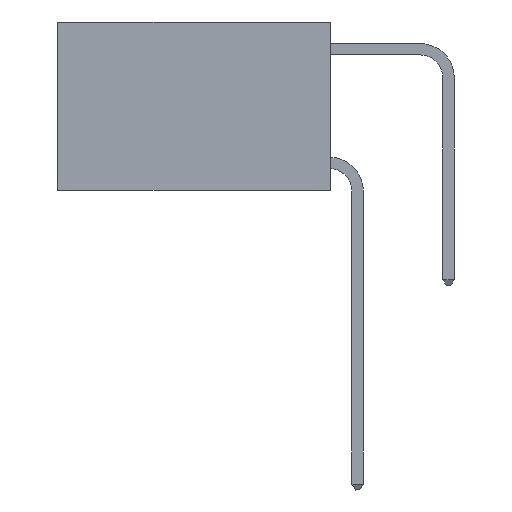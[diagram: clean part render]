
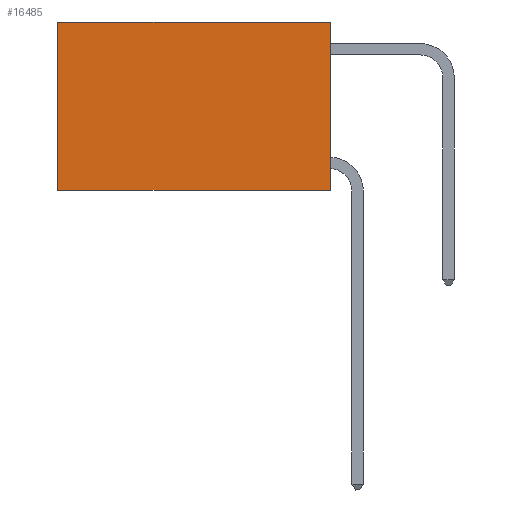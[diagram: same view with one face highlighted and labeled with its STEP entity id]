
A CAD part, left-side view. The second image highlights one B-rep face of the part: STEP entity #16485.
In plain terms, the highlighted planar face has unit normal (-1, 0, 0).
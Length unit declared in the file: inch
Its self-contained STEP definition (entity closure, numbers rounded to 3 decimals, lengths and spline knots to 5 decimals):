
#1286 = LINE ( 'NONE', #7868, #14220 ) ;
#1304 = PLANE ( 'NONE',  #7939 ) ;
#2613 = ORIENTED_EDGE ( 'NONE', *, *, #19795, .T. ) ;
#2713 = VERTEX_POINT ( 'NONE', #18414 ) ;
#2981 = FACE_OUTER_BOUND ( 'NONE', #11656, .T. ) ;
#2998 = DIRECTION ( 'NONE',  ( 0., 0., -1. ) ) ;
#3910 = CARTESIAN_POINT ( 'NONE',  ( 0.2625, 0., 0. ) ) ;
#4216 = EDGE_CURVE ( 'NONE', #17136, #19659, #1286, .T. ) ;
#4768 = CARTESIAN_POINT ( 'NONE',  ( 0.2625, 0., 0. ) ) ;
#4852 = DIRECTION ( 'NONE',  ( 0., 1., 0. ) ) ;
#4971 = CARTESIAN_POINT ( 'NONE',  ( 0.2625, 0.6, -0.37 ) ) ;
#5372 = LINE ( 'NONE', #8292, #13201 ) ;
#5967 = CARTESIAN_POINT ( 'NONE',  ( 0.2625, 0., -0.37 ) ) ;
#7577 = DIRECTION ( 'NONE',  ( 0., 0., -1. ) ) ;
#7868 = CARTESIAN_POINT ( 'NONE',  ( 0.2625, 0., -0.37 ) ) ;
#7939 = AXIS2_PLACEMENT_3D ( 'NONE', #9346, #9450, #17512 ) ;
#8292 = CARTESIAN_POINT ( 'NONE',  ( 0.2625, 0.6, 0. ) ) ;
#9286 = VERTEX_POINT ( 'NONE', #14115 ) ;
#9346 = CARTESIAN_POINT ( 'NONE',  ( 0.2625, 0., 0. ) ) ;
#9450 = DIRECTION ( 'NONE',  ( 1., 0., 0. ) ) ;
#10921 = LINE ( 'NONE', #4768, #12618 ) ;
#11656 = EDGE_LOOP ( 'NONE', ( #16651, #12551, #17607, #2613 ) ) ;
#12551 = ORIENTED_EDGE ( 'NONE', *, *, #4216, .F. ) ;
#12618 = VECTOR ( 'NONE', #7577, 39.37008 ) ;
#13201 = VECTOR ( 'NONE', #2998, 39.37008 ) ;
#14115 = CARTESIAN_POINT ( 'NONE',  ( 0.2625, 0., 0. ) ) ;
#14220 = VECTOR ( 'NONE', #4852, 39.37008 ) ;
#15219 = VECTOR ( 'NONE', #18121, 39.37008 ) ;
#16485 = ADVANCED_FACE ( 'NONE', ( #2981 ), #1304, .F. ) ;
#16486 = EDGE_CURVE ( 'NONE', #9286, #17136, #10921, .T. ) ;
#16651 = ORIENTED_EDGE ( 'NONE', *, *, #19723, .T. ) ;
#17136 = VERTEX_POINT ( 'NONE', #5967 ) ;
#17512 = DIRECTION ( 'NONE',  ( 0., 0., -1. ) ) ;
#17607 = ORIENTED_EDGE ( 'NONE', *, *, #16486, .F. ) ;
#18121 = DIRECTION ( 'NONE',  ( 0., 1., 0. ) ) ;
#18329 = LINE ( 'NONE', #3910, #15219 ) ;
#18414 = CARTESIAN_POINT ( 'NONE',  ( 0.2625, 0.6, 0. ) ) ;
#19659 = VERTEX_POINT ( 'NONE', #4971 ) ;
#19723 = EDGE_CURVE ( 'NONE', #2713, #19659, #5372, .T. ) ;
#19795 = EDGE_CURVE ( 'NONE', #9286, #2713, #18329, .T. ) ;
